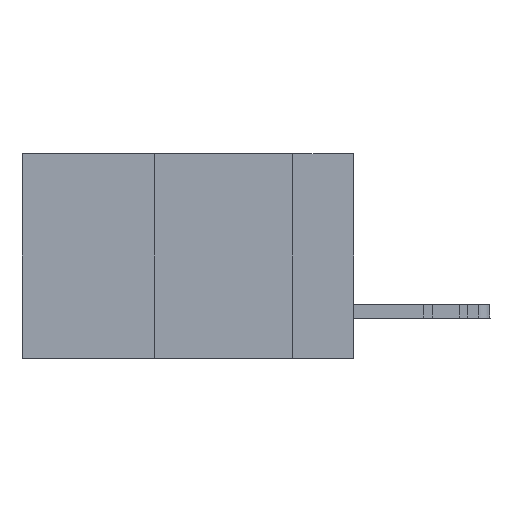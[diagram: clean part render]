
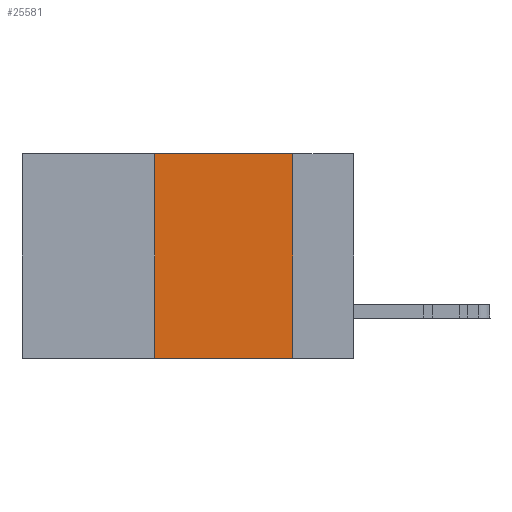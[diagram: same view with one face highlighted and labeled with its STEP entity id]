
A CAD part, left-side view. The second image highlights one B-rep face of the part: STEP entity #25581.
In plain terms, the highlighted planar face has unit normal (-1, 0, 0).
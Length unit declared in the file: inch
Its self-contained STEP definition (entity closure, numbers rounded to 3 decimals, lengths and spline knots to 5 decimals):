
#240 = LINE ( 'NONE', #15146, #32498 ) ;
#2461 = DIRECTION ( 'NONE',  ( 0., 0., -1. ) ) ;
#3314 = PLANE ( 'NONE',  #19647 ) ;
#3405 = LINE ( 'NONE', #30440, #27340 ) ;
#4398 = VERTEX_POINT ( 'NONE', #7866 ) ;
#4836 = CARTESIAN_POINT ( 'NONE',  ( 0., 0.36, 0. ) ) ;
#6455 = DIRECTION ( 'NONE',  ( 1., 0., 0. ) ) ;
#7866 = CARTESIAN_POINT ( 'NONE',  ( 0., 0.11, 0. ) ) ;
#8310 = VERTEX_POINT ( 'NONE', #38469 ) ;
#8956 = DIRECTION ( 'NONE',  ( 0., -1., 0. ) ) ;
#9238 = CARTESIAN_POINT ( 'NONE',  ( 0., 0.6, 0. ) ) ;
#9427 = CARTESIAN_POINT ( 'NONE',  ( 0., 0.6, 0. ) ) ;
#12411 = DIRECTION ( 'NONE',  ( 0., -1., 0. ) ) ;
#13040 = LINE ( 'NONE', #9238, #36865 ) ;
#13411 = ORIENTED_EDGE ( 'NONE', *, *, #39314, .F. ) ;
#15146 = CARTESIAN_POINT ( 'NONE',  ( 0., 0.6, -0.37 ) ) ;
#15659 = VERTEX_POINT ( 'NONE', #4836 ) ;
#16496 = EDGE_CURVE ( 'NONE', #32648, #8310, #240, .T. ) ;
#16648 = ORIENTED_EDGE ( 'NONE', *, *, #16496, .T. ) ;
#19644 = CARTESIAN_POINT ( 'NONE',  ( 0., 0.36, 0. ) ) ;
#19647 = AXIS2_PLACEMENT_3D ( 'NONE', #9427, #6455, #28286 ) ;
#19649 = LINE ( 'NONE', #19644, #35251 ) ;
#22750 = DIRECTION ( 'NONE',  ( 0., 0., 1. ) ) ;
#24724 = EDGE_LOOP ( 'NONE', ( #27744, #13411, #27752, #16648 ) ) ;
#25581 = ADVANCED_FACE ( 'NONE', ( #37334 ), #3314, .F. ) ;
#27340 = VECTOR ( 'NONE', #2461, 39.37008 ) ;
#27744 = ORIENTED_EDGE ( 'NONE', *, *, #29821, .F. ) ;
#27752 = ORIENTED_EDGE ( 'NONE', *, *, #31929, .F. ) ;
#28286 = DIRECTION ( 'NONE',  ( 0., 0., -1. ) ) ;
#29821 = EDGE_CURVE ( 'NONE', #4398, #8310, #3405, .T. ) ;
#30440 = CARTESIAN_POINT ( 'NONE',  ( 0., 0.11, 0. ) ) ;
#31929 = EDGE_CURVE ( 'NONE', #32648, #15659, #19649, .T. ) ;
#32498 = VECTOR ( 'NONE', #8956, 39.37008 ) ;
#32648 = VERTEX_POINT ( 'NONE', #34613 ) ;
#34613 = CARTESIAN_POINT ( 'NONE',  ( 0., 0.36, -0.37 ) ) ;
#35251 = VECTOR ( 'NONE', #22750, 39.37008 ) ;
#36865 = VECTOR ( 'NONE', #12411, 39.37008 ) ;
#37334 = FACE_OUTER_BOUND ( 'NONE', #24724, .T. ) ;
#38469 = CARTESIAN_POINT ( 'NONE',  ( 0., 0.11, -0.37 ) ) ;
#39314 = EDGE_CURVE ( 'NONE', #15659, #4398, #13040, .T. ) ;
